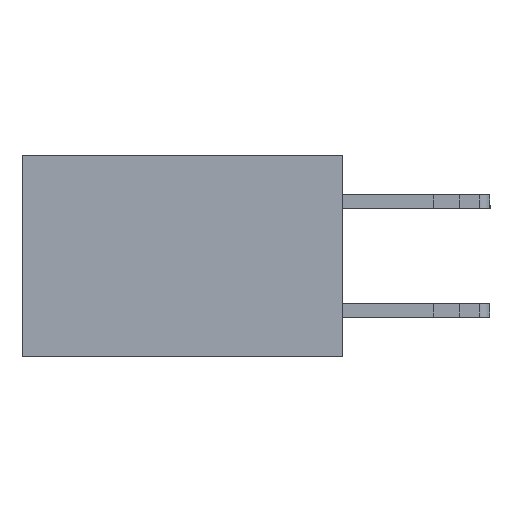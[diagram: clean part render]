
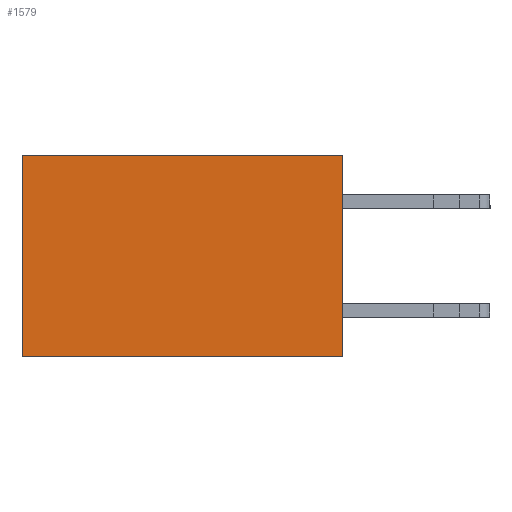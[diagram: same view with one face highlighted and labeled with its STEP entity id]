
A CAD part, left-side view. The second image highlights one B-rep face of the part: STEP entity #1579.
In plain terms, the highlighted planar face has unit normal (-1, 0, 0).
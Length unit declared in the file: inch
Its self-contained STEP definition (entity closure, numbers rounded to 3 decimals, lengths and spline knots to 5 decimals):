
#1307 = DIRECTION ( 'NONE',  ( 0., 0., -1. ) ) ;
#1579 = ADVANCED_FACE ( 'NONE', ( #4361 ), #14302, .F. ) ;
#2997 = VECTOR ( 'NONE', #10772, 39.37008 ) ;
#3464 = EDGE_CURVE ( 'NONE', #17868, #28235, #31115, .T. ) ;
#4162 = ORIENTED_EDGE ( 'NONE', *, *, #17551, .F. ) ;
#4361 = FACE_OUTER_BOUND ( 'NONE', #7147, .T. ) ;
#5391 = LINE ( 'NONE', #9039, #27381 ) ;
#7147 = EDGE_LOOP ( 'NONE', ( #23735, #4162, #29211, #16666 ) ) ;
#8188 = CARTESIAN_POINT ( 'NONE',  ( 0.277, 0., -0.37 ) ) ;
#9039 = CARTESIAN_POINT ( 'NONE',  ( 0.277, 0.59, -0.37 ) ) ;
#9075 = DIRECTION ( 'NONE',  ( 0., 0., -1. ) ) ;
#10772 = DIRECTION ( 'NONE',  ( 0., 1., 0. ) ) ;
#11882 = EDGE_CURVE ( 'NONE', #28235, #13699, #5391, .T. ) ;
#12066 = CARTESIAN_POINT ( 'NONE',  ( 0.277, 0., -0.37 ) ) ;
#13699 = VERTEX_POINT ( 'NONE', #30344 ) ;
#13990 = DIRECTION ( 'NONE',  ( 0., 1., 0. ) ) ;
#14302 = PLANE ( 'NONE',  #26645 ) ;
#16401 = DIRECTION ( 'NONE',  ( 1., 0., 0. ) ) ;
#16559 = DIRECTION ( 'NONE',  ( 0., 0., -1. ) ) ;
#16654 = CARTESIAN_POINT ( 'NONE',  ( 0.277, 0.59, 0. ) ) ;
#16666 = ORIENTED_EDGE ( 'NONE', *, *, #3464, .T. ) ;
#16711 = CARTESIAN_POINT ( 'NONE',  ( 0.277, 0., -0.37 ) ) ;
#17551 = EDGE_CURVE ( 'NONE', #19135, #13699, #23400, .T. ) ;
#17868 = VERTEX_POINT ( 'NONE', #24462 ) ;
#17900 = VECTOR ( 'NONE', #13990, 39.37008 ) ;
#19135 = VERTEX_POINT ( 'NONE', #21962 ) ;
#19888 = EDGE_CURVE ( 'NONE', #17868, #19135, #28727, .T. ) ;
#21962 = CARTESIAN_POINT ( 'NONE',  ( 0.277, 0., -0.37 ) ) ;
#22091 = VECTOR ( 'NONE', #9075, 39.37008 ) ;
#22137 = CARTESIAN_POINT ( 'NONE',  ( 0.277, 0., 0. ) ) ;
#23400 = LINE ( 'NONE', #8188, #2997 ) ;
#23735 = ORIENTED_EDGE ( 'NONE', *, *, #11882, .T. ) ;
#24462 = CARTESIAN_POINT ( 'NONE',  ( 0.277, 0., 0. ) ) ;
#26645 = AXIS2_PLACEMENT_3D ( 'NONE', #12066, #16401, #16559 ) ;
#27381 = VECTOR ( 'NONE', #1307, 39.37008 ) ;
#28235 = VERTEX_POINT ( 'NONE', #16654 ) ;
#28727 = LINE ( 'NONE', #16711, #22091 ) ;
#29211 = ORIENTED_EDGE ( 'NONE', *, *, #19888, .F. ) ;
#30344 = CARTESIAN_POINT ( 'NONE',  ( 0.277, 0.59, -0.37 ) ) ;
#31115 = LINE ( 'NONE', #22137, #17900 ) ;
